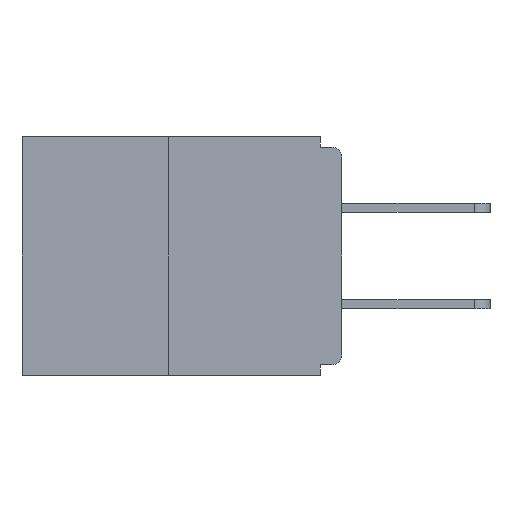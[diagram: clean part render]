
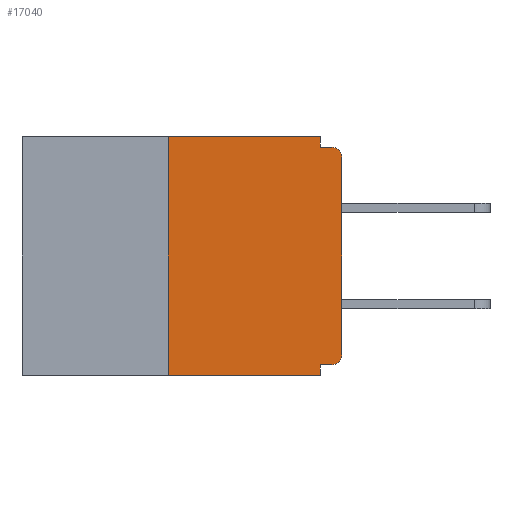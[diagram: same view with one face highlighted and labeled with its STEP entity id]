
A CAD part, left-side view. The second image highlights one B-rep face of the part: STEP entity #17040.
In plain terms, the highlighted planar face has unit normal (-1, 0, 0).
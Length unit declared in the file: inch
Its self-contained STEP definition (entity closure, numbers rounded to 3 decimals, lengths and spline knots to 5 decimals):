
#40 = CARTESIAN_POINT ( 'NONE',  ( 0., 0.015, -0.03 ) ) ;
#62 = ORIENTED_EDGE ( 'NONE', *, *, #19354, .F. ) ;
#226 = DIRECTION ( 'NONE',  ( 0., 0., 1. ) ) ;
#548 = DIRECTION ( 'NONE',  ( 0., 0., -1. ) ) ;
#729 = AXIS2_PLACEMENT_3D ( 'NONE', #40, #4347, #16305 ) ;
#913 = CARTESIAN_POINT ( 'NONE',  ( 0., 0.015, -0.328 ) ) ;
#971 = CARTESIAN_POINT ( 'NONE',  ( 0., 0.25, -0.343 ) ) ;
#1164 = EDGE_CURVE ( 'NONE', #20181, #8536, #4686, .T. ) ;
#1667 = DIRECTION ( 'NONE',  ( 0., -1., 0. ) ) ;
#1944 = EDGE_CURVE ( 'NONE', #12095, #8588, #2758, .T. ) ;
#2265 = VERTEX_POINT ( 'NONE', #3682 ) ;
#2467 = CARTESIAN_POINT ( 'NONE',  ( 0., 0.031, -0.328 ) ) ;
#2758 = LINE ( 'NONE', #24282, #4344 ) ;
#2852 = ORIENTED_EDGE ( 'NONE', *, *, #20153, .F. ) ;
#3587 = CARTESIAN_POINT ( 'NONE',  ( 0., 0.031, -0.343 ) ) ;
#3682 = CARTESIAN_POINT ( 'NONE',  ( 0., 0.031, -0.015 ) ) ;
#3913 = VERTEX_POINT ( 'NONE', #2467 ) ;
#4344 = VECTOR ( 'NONE', #9811, 39.37008 ) ;
#4347 = DIRECTION ( 'NONE',  ( -1., 0., 0. ) ) ;
#4404 = VERTEX_POINT ( 'NONE', #6512 ) ;
#4503 = DIRECTION ( 'NONE',  ( -1., 0., 0. ) ) ;
#4686 = CIRCLE ( 'NONE', #23927, 0.015 ) ;
#4814 = AXIS2_PLACEMENT_3D ( 'NONE', #23840, #23661, #13865 ) ;
#4991 = LINE ( 'NONE', #8337, #14465 ) ;
#5327 = EDGE_CURVE ( 'NONE', #5854, #4404, #19664, .T. ) ;
#5823 = LINE ( 'NONE', #14233, #7098 ) ;
#5854 = VERTEX_POINT ( 'NONE', #16594 ) ;
#6289 = EDGE_CURVE ( 'NONE', #12095, #5854, #19947, .T. ) ;
#6329 = ORIENTED_EDGE ( 'NONE', *, *, #23464, .F. ) ;
#6512 = CARTESIAN_POINT ( 'NONE',  ( 0., 0.031, 0. ) ) ;
#6636 = CARTESIAN_POINT ( 'NONE',  ( 0., 0.031, 0. ) ) ;
#6660 = LINE ( 'NONE', #24431, #21820 ) ;
#6853 = CARTESIAN_POINT ( 'NONE',  ( 0., 0.015, -0.015 ) ) ;
#7098 = VECTOR ( 'NONE', #14323, 39.37008 ) ;
#8332 = CARTESIAN_POINT ( 'NONE',  ( 0., 0., -0.03 ) ) ;
#8337 = CARTESIAN_POINT ( 'NONE',  ( 0., 0., 0. ) ) ;
#8536 = VERTEX_POINT ( 'NONE', #9939 ) ;
#8588 = VERTEX_POINT ( 'NONE', #3587 ) ;
#8863 = EDGE_LOOP ( 'NONE', ( #12260, #20505, #19833, #6329, #62, #13278, #13165, #11309, #24943, #2852 ) ) ;
#8944 = EDGE_CURVE ( 'NONE', #2265, #19513, #5823, .T. ) ;
#9139 = VERTEX_POINT ( 'NONE', #8332 ) ;
#9811 = DIRECTION ( 'NONE',  ( 0., -1., 0. ) ) ;
#9939 = CARTESIAN_POINT ( 'NONE',  ( 0., 0., -0.313 ) ) ;
#11158 = LINE ( 'NONE', #6636, #20019 ) ;
#11309 = ORIENTED_EDGE ( 'NONE', *, *, #25045, .T. ) ;
#11601 = CARTESIAN_POINT ( 'NONE',  ( 0., 0.25, 0. ) ) ;
#12075 = CARTESIAN_POINT ( 'NONE',  ( 0., 0.46, 0. ) ) ;
#12095 = VERTEX_POINT ( 'NONE', #971 ) ;
#12260 = ORIENTED_EDGE ( 'NONE', *, *, #5327, .F. ) ;
#13165 = ORIENTED_EDGE ( 'NONE', *, *, #14975, .T. ) ;
#13278 = ORIENTED_EDGE ( 'NONE', *, *, #1164, .T. ) ;
#13340 = VECTOR ( 'NONE', #1667, 39.37008 ) ;
#13640 = DIRECTION ( 'NONE',  ( 0., 0., 1. ) ) ;
#13865 = DIRECTION ( 'NONE',  ( 0., 0., -1. ) ) ;
#14166 = LINE ( 'NONE', #21924, #24600 ) ;
#14233 = CARTESIAN_POINT ( 'NONE',  ( 0., 0., -0.015 ) ) ;
#14323 = DIRECTION ( 'NONE',  ( 0., -1., 0. ) ) ;
#14465 = VECTOR ( 'NONE', #226, 39.37008 ) ;
#14975 = EDGE_CURVE ( 'NONE', #8536, #9139, #4991, .T. ) ;
#16305 = DIRECTION ( 'NONE',  ( 0., 0., -1. ) ) ;
#16568 = DIRECTION ( 'NONE',  ( 0., 0., -1. ) ) ;
#16594 = CARTESIAN_POINT ( 'NONE',  ( 0., 0.25, 0. ) ) ;
#17040 = ADVANCED_FACE ( 'NONE', ( #17539 ), #21815, .F. ) ;
#17130 = VECTOR ( 'NONE', #13640, 39.37008 ) ;
#17539 = FACE_OUTER_BOUND ( 'NONE', #8863, .T. ) ;
#18213 = CIRCLE ( 'NONE', #729, 0.015 ) ;
#19354 = EDGE_CURVE ( 'NONE', #20181, #3913, #6660, .T. ) ;
#19513 = VERTEX_POINT ( 'NONE', #6853 ) ;
#19664 = LINE ( 'NONE', #12075, #13340 ) ;
#19833 = ORIENTED_EDGE ( 'NONE', *, *, #1944, .T. ) ;
#19947 = LINE ( 'NONE', #11601, #17130 ) ;
#20019 = VECTOR ( 'NONE', #16568, 39.37008 ) ;
#20153 = EDGE_CURVE ( 'NONE', #4404, #2265, #11158, .T. ) ;
#20181 = VERTEX_POINT ( 'NONE', #913 ) ;
#20391 = DIRECTION ( 'NONE',  ( 0., 1., 0. ) ) ;
#20505 = ORIENTED_EDGE ( 'NONE', *, *, #6289, .F. ) ;
#21012 = CARTESIAN_POINT ( 'NONE',  ( 0., 0.015, -0.313 ) ) ;
#21815 = PLANE ( 'NONE',  #4814 ) ;
#21820 = VECTOR ( 'NONE', #20391, 39.37008 ) ;
#21924 = CARTESIAN_POINT ( 'NONE',  ( 0., 0.031, -0.343 ) ) ;
#23464 = EDGE_CURVE ( 'NONE', #3913, #8588, #14166, .T. ) ;
#23661 = DIRECTION ( 'NONE',  ( 1., 0., 0. ) ) ;
#23840 = CARTESIAN_POINT ( 'NONE',  ( 0., 0.46, 0. ) ) ;
#23927 = AXIS2_PLACEMENT_3D ( 'NONE', #21012, #4503, #548 ) ;
#24282 = CARTESIAN_POINT ( 'NONE',  ( 0., 0.46, -0.343 ) ) ;
#24431 = CARTESIAN_POINT ( 'NONE',  ( 0., 0., -0.328 ) ) ;
#24600 = VECTOR ( 'NONE', #25978, 39.37008 ) ;
#24943 = ORIENTED_EDGE ( 'NONE', *, *, #8944, .F. ) ;
#25045 = EDGE_CURVE ( 'NONE', #9139, #19513, #18213, .T. ) ;
#25978 = DIRECTION ( 'NONE',  ( 0., 0., -1. ) ) ;
